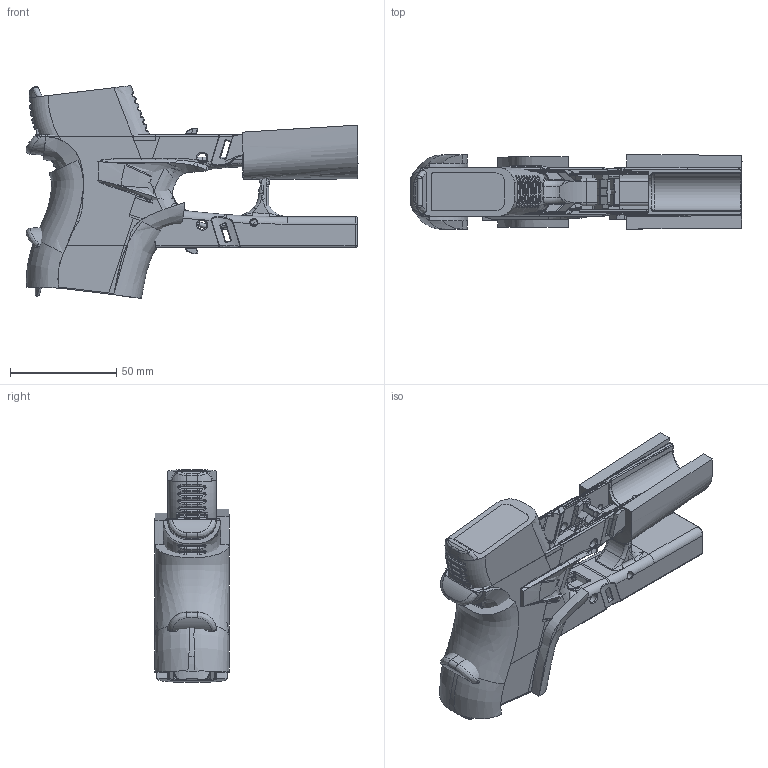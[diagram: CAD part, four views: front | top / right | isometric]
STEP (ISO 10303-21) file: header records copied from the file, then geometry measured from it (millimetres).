
FILE_DESCRIPTION(/* description */ ('Unknown'),/* implementation_level */ '2;1');
FILE_NAME(/* name */ '34 chairmanwon',/* time_stamp */ '2022-01-12T06:00:17-05:00',/* author */ ('Unknown'),/* organization */ ('Unknown'),/* preprocessor_version */ 'ST-DEVELOPER v16.7',/* originating_system */ 'DEX',/* authorisation */ $);
FILE_SCHEMA (('AUTOMOTIVE_DESIGN {1 0 10303 214 3 1 1}'));
Products named in the file (1): Frame
Bounding box: 156.2 x 35 x 100.08 mm (x, y, z)
Volume: 191211.9 mm3; surface area: 127604.9 mm2
Topology: 11 solids, 11 shells, 3360 faces, 8656 edges, 5145 vertices
Faces by surface type: bspline 1212, cylinder 1037, plane 650, torus 294, sphere 104, cone 63
Full cylindrical faces by diameter (mm): 3.05 x6, 3.3 x6, 3.5 x3, 4.25 x6
Entity records: 162190 total; most frequent: CARTESIAN_POINT 85742, ORIENTED_EDGE 16918, DIRECTION 11163, EDGE_CURVE 8459, VERTEX_POINT 5118, AXIS2_PLACEMENT_3D 4300, B_SPLINE_CURVE_WITH_KNOTS 3736, EDGE_LOOP 3439
